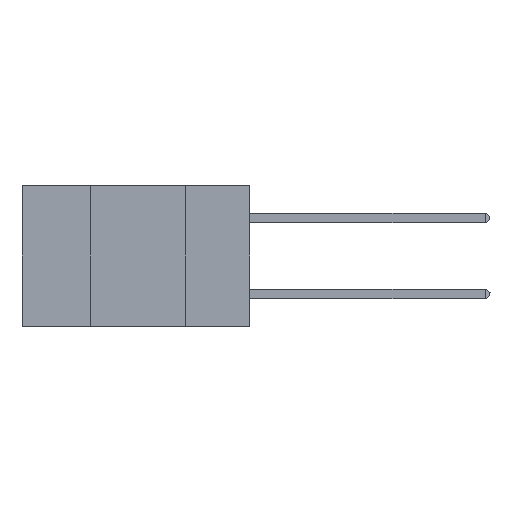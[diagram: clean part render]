
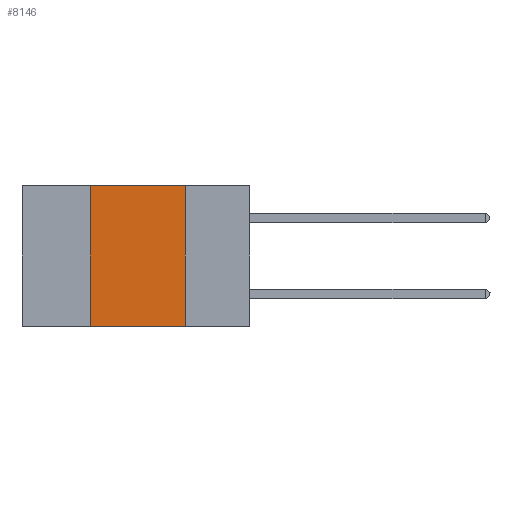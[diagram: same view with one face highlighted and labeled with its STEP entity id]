
A CAD part, left-side view. The second image highlights one B-rep face of the part: STEP entity #8146.
In plain terms, the highlighted planar face has unit normal (-1, 0, 0).
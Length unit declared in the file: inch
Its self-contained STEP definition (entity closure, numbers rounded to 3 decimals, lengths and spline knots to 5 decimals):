
#338 = ORIENTED_EDGE ( 'NONE', *, *, #2192, .F. ) ;
#1913 = VERTEX_POINT ( 'NONE', #20906 ) ;
#2095 = VERTEX_POINT ( 'NONE', #6852 ) ;
#2192 = EDGE_CURVE ( 'NONE', #2095, #1913, #25203, .T. ) ;
#3226 = DIRECTION ( 'NONE',  ( 0., -1., 0. ) ) ;
#4381 = VECTOR ( 'NONE', #26257, 39.37008 ) ;
#5613 = LINE ( 'NONE', #19074, #25254 ) ;
#6499 = DIRECTION ( 'NONE',  ( 0., -1., 0. ) ) ;
#6852 = CARTESIAN_POINT ( 'NONE',  ( 0., 0.42, -0.37 ) ) ;
#7552 = ORIENTED_EDGE ( 'NONE', *, *, #8175, .F. ) ;
#8146 = ADVANCED_FACE ( 'NONE', ( #22107 ), #24237, .F. ) ;
#8175 = EDGE_CURVE ( 'NONE', #18028, #15593, #17508, .T. ) ;
#9619 = CARTESIAN_POINT ( 'NONE',  ( 0., 0.17, 0. ) ) ;
#10891 = EDGE_LOOP ( 'NONE', ( #7552, #16857, #338, #20883 ) ) ;
#11401 = DIRECTION ( 'NONE',  ( 0., 0., 1. ) ) ;
#11481 = AXIS2_PLACEMENT_3D ( 'NONE', #20142, #26352, #15915 ) ;
#11887 = CARTESIAN_POINT ( 'NONE',  ( 0., 0.6, 0. ) ) ;
#15554 = CARTESIAN_POINT ( 'NONE',  ( 0., 0.42, 0. ) ) ;
#15593 = VERTEX_POINT ( 'NONE', #26310 ) ;
#15705 = VECTOR ( 'NONE', #11401, 39.37008 ) ;
#15915 = DIRECTION ( 'NONE',  ( 0., 0., -1. ) ) ;
#16857 = ORIENTED_EDGE ( 'NONE', *, *, #22268, .F. ) ;
#17124 = VECTOR ( 'NONE', #3226, 39.37008 ) ;
#17508 = LINE ( 'NONE', #9619, #4381 ) ;
#18028 = VERTEX_POINT ( 'NONE', #18314 ) ;
#18314 = CARTESIAN_POINT ( 'NONE',  ( 0., 0.17, 0. ) ) ;
#19074 = CARTESIAN_POINT ( 'NONE',  ( 0., 0.6, -0.37 ) ) ;
#19093 = LINE ( 'NONE', #11887, #17124 ) ;
#20142 = CARTESIAN_POINT ( 'NONE',  ( 0., 0.6, 0. ) ) ;
#20883 = ORIENTED_EDGE ( 'NONE', *, *, #22545, .T. ) ;
#20906 = CARTESIAN_POINT ( 'NONE',  ( 0., 0.42, 0. ) ) ;
#22107 = FACE_OUTER_BOUND ( 'NONE', #10891, .T. ) ;
#22268 = EDGE_CURVE ( 'NONE', #1913, #18028, #19093, .T. ) ;
#22545 = EDGE_CURVE ( 'NONE', #2095, #15593, #5613, .T. ) ;
#24237 = PLANE ( 'NONE',  #11481 ) ;
#25203 = LINE ( 'NONE', #15554, #15705 ) ;
#25254 = VECTOR ( 'NONE', #6499, 39.37008 ) ;
#26257 = DIRECTION ( 'NONE',  ( 0., 0., -1. ) ) ;
#26310 = CARTESIAN_POINT ( 'NONE',  ( 0., 0.17, -0.37 ) ) ;
#26352 = DIRECTION ( 'NONE',  ( 1., 0., 0. ) ) ;
